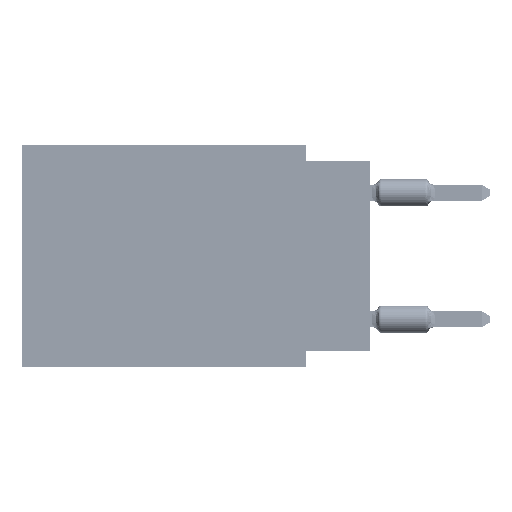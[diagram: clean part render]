
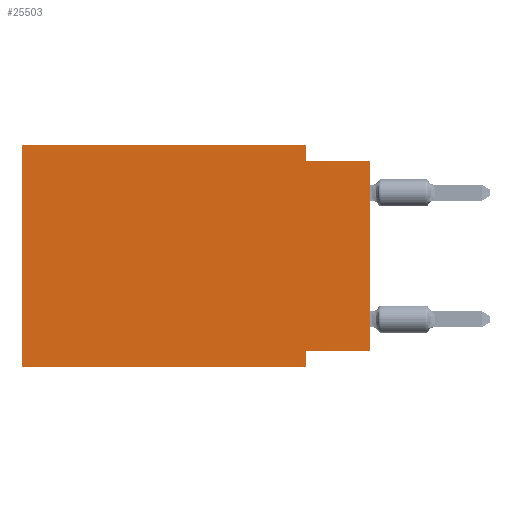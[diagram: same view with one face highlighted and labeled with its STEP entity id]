
A CAD part, left-side view. The second image highlights one B-rep face of the part: STEP entity #25503.
In plain terms, the highlighted planar face has unit normal (-1, 0, 0).
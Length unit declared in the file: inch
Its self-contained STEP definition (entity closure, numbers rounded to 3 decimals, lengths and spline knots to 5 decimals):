
#2631 = VECTOR ( 'NONE', #58971, 39.37008 ) ;
#3021 = VECTOR ( 'NONE', #44971, 39.37008 ) ;
#3510 = DIRECTION ( 'NONE',  ( 0., 0., -1. ) ) ;
#5521 = EDGE_CURVE ( 'NONE', #59092, #19538, #20331, .T. ) ;
#6116 = VERTEX_POINT ( 'NONE', #57646 ) ;
#6966 = DIRECTION ( 'NONE',  ( 0., -1., 0. ) ) ;
#8022 = VERTEX_POINT ( 'NONE', #40063 ) ;
#9311 = VECTOR ( 'NONE', #6966, 39.37008 ) ;
#11466 = VECTOR ( 'NONE', #66766, 39.37008 ) ;
#11698 = LINE ( 'NONE', #33025, #55419 ) ;
#13141 = LINE ( 'NONE', #24325, #3021 ) ;
#13654 = CARTESIAN_POINT ( 'NONE',  ( 0., 0.55, 0. ) ) ;
#15508 = ORIENTED_EDGE ( 'NONE', *, *, #43082, .T. ) ;
#17168 = CARTESIAN_POINT ( 'NONE',  ( 0., 0.1, 0. ) ) ;
#17458 = CARTESIAN_POINT ( 'NONE',  ( 0., 0.55, 0. ) ) ;
#17509 = DIRECTION ( 'NONE',  ( 0., 0., -1. ) ) ;
#18178 = LINE ( 'NONE', #24110, #11466 ) ;
#18530 = ORIENTED_EDGE ( 'NONE', *, *, #28319, .F. ) ;
#19538 = VERTEX_POINT ( 'NONE', #34156 ) ;
#19686 = DIRECTION ( 'NONE',  ( 0., 0., 1. ) ) ;
#19975 = ORIENTED_EDGE ( 'NONE', *, *, #42056, .F. ) ;
#20331 = LINE ( 'NONE', #66863, #33906 ) ;
#24110 = CARTESIAN_POINT ( 'NONE',  ( 0., 0., -0.025 ) ) ;
#24325 = CARTESIAN_POINT ( 'NONE',  ( 0., 0.55, 0. ) ) ;
#25150 = VECTOR ( 'NONE', #17509, 39.37008 ) ;
#25503 = ADVANCED_FACE ( 'NONE', ( #35685 ), #29391, .F. ) ;
#27805 = ORIENTED_EDGE ( 'NONE', *, *, #54626, .F. ) ;
#28319 = EDGE_CURVE ( 'NONE', #55648, #57052, #65362, .T. ) ;
#29391 = PLANE ( 'NONE',  #59074 ) ;
#31591 = EDGE_CURVE ( 'NONE', #8022, #6116, #11698, .T. ) ;
#33025 = CARTESIAN_POINT ( 'NONE',  ( 0., 0., 0. ) ) ;
#33518 = EDGE_LOOP ( 'NONE', ( #58762, #45552, #19975, #18530, #41585, #15508, #52724, #27805 ) ) ;
#33906 = VECTOR ( 'NONE', #35737, 39.37008 ) ;
#34156 = CARTESIAN_POINT ( 'NONE',  ( 0., 0.1, -0.35 ) ) ;
#34989 = DIRECTION ( 'NONE',  ( 1., 0., 0. ) ) ;
#35685 = FACE_OUTER_BOUND ( 'NONE', #33518, .T. ) ;
#35737 = DIRECTION ( 'NONE',  ( 0., 0., -1. ) ) ;
#35910 = CARTESIAN_POINT ( 'NONE',  ( 0., 0.1, -0.325 ) ) ;
#37817 = LINE ( 'NONE', #17168, #25150 ) ;
#38290 = CARTESIAN_POINT ( 'NONE',  ( 0., 0.1, -0.025 ) ) ;
#39498 = CARTESIAN_POINT ( 'NONE',  ( 0., 0.55, -0.35 ) ) ;
#40063 = CARTESIAN_POINT ( 'NONE',  ( 0., 0., -0.325 ) ) ;
#40663 = DIRECTION ( 'NONE',  ( 0., -1., 0. ) ) ;
#41585 = ORIENTED_EDGE ( 'NONE', *, *, #60237, .F. ) ;
#42056 = EDGE_CURVE ( 'NONE', #57052, #65869, #37817, .T. ) ;
#43082 = EDGE_CURVE ( 'NONE', #58590, #19538, #66897, .T. ) ;
#44971 = DIRECTION ( 'NONE',  ( 0., 0., 1. ) ) ;
#45552 = ORIENTED_EDGE ( 'NONE', *, *, #52167, .F. ) ;
#47443 = CARTESIAN_POINT ( 'NONE',  ( 0., 0., -0.325 ) ) ;
#52167 = EDGE_CURVE ( 'NONE', #65869, #6116, #18178, .T. ) ;
#52180 = CARTESIAN_POINT ( 'NONE',  ( 0., 0.55, -0.35 ) ) ;
#52724 = ORIENTED_EDGE ( 'NONE', *, *, #5521, .F. ) ;
#54626 = EDGE_CURVE ( 'NONE', #8022, #59092, #58623, .T. ) ;
#55419 = VECTOR ( 'NONE', #19686, 39.37008 ) ;
#55648 = VERTEX_POINT ( 'NONE', #56211 ) ;
#56211 = CARTESIAN_POINT ( 'NONE',  ( 0., 0.55, 0. ) ) ;
#57052 = VERTEX_POINT ( 'NONE', #61931 ) ;
#57646 = CARTESIAN_POINT ( 'NONE',  ( 0., 0., -0.025 ) ) ;
#58590 = VERTEX_POINT ( 'NONE', #39498 ) ;
#58623 = LINE ( 'NONE', #47443, #2631 ) ;
#58762 = ORIENTED_EDGE ( 'NONE', *, *, #31591, .T. ) ;
#58971 = DIRECTION ( 'NONE',  ( 0., 1., 0. ) ) ;
#59074 = AXIS2_PLACEMENT_3D ( 'NONE', #13654, #34989, #3510 ) ;
#59092 = VERTEX_POINT ( 'NONE', #35910 ) ;
#60237 = EDGE_CURVE ( 'NONE', #58590, #55648, #13141, .T. ) ;
#61931 = CARTESIAN_POINT ( 'NONE',  ( 0., 0.1, 0. ) ) ;
#65362 = LINE ( 'NONE', #17458, #9311 ) ;
#65869 = VERTEX_POINT ( 'NONE', #38290 ) ;
#66526 = VECTOR ( 'NONE', #40663, 39.37008 ) ;
#66766 = DIRECTION ( 'NONE',  ( 0., -1., 0. ) ) ;
#66863 = CARTESIAN_POINT ( 'NONE',  ( 0., 0.1, -0.35 ) ) ;
#66897 = LINE ( 'NONE', #52180, #66526 ) ;
